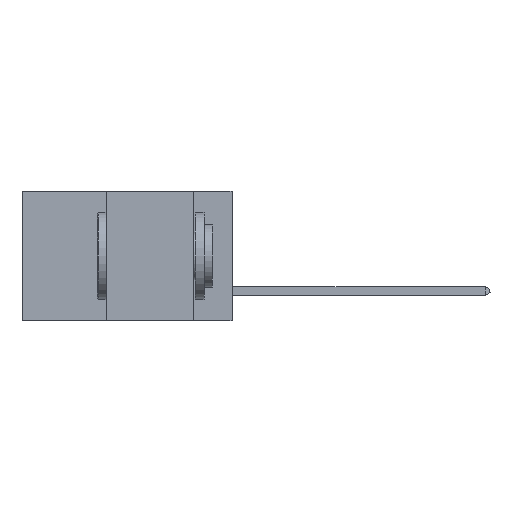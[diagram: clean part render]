
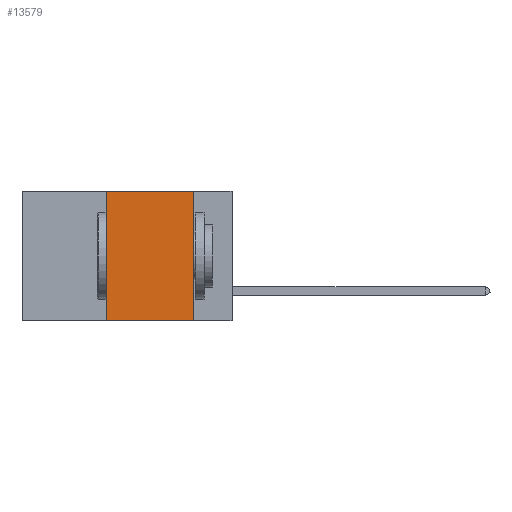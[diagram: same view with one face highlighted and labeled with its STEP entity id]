
A CAD part, left-side view. The second image highlights one B-rep face of the part: STEP entity #13579.
In plain terms, the highlighted planar face has unit normal (-1, 0, 0).
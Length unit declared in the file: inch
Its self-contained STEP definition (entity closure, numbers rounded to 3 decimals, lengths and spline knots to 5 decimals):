
#772 = VECTOR ( 'NONE', #7230, 39.37008 ) ;
#856 = EDGE_CURVE ( 'NONE', #14611, #11134, #8960, .T. ) ;
#1197 = VECTOR ( 'NONE', #9243, 39.37008 ) ;
#1568 = CARTESIAN_POINT ( 'NONE',  ( 0., 0.36, 0. ) ) ;
#1757 = CARTESIAN_POINT ( 'NONE',  ( 0., 0.36, -0.37 ) ) ;
#3604 = ORIENTED_EDGE ( 'NONE', *, *, #4131, .F. ) ;
#4131 = EDGE_CURVE ( 'NONE', #13491, #6629, #10320, .T. ) ;
#4282 = CARTESIAN_POINT ( 'NONE',  ( 0., 0.11, 0. ) ) ;
#4395 = CARTESIAN_POINT ( 'NONE',  ( 0., 0.6, -0.37 ) ) ;
#5053 = DIRECTION ( 'NONE',  ( 0., 0., -1. ) ) ;
#5174 = PLANE ( 'NONE',  #9892 ) ;
#5248 = LINE ( 'NONE', #4395, #8461 ) ;
#6492 = CARTESIAN_POINT ( 'NONE',  ( 0., 0.11, -0.37 ) ) ;
#6629 = VERTEX_POINT ( 'NONE', #1568 ) ;
#7043 = ORIENTED_EDGE ( 'NONE', *, *, #856, .F. ) ;
#7155 = EDGE_LOOP ( 'NONE', ( #7043, #13003, #3604, #12993 ) ) ;
#7230 = DIRECTION ( 'NONE',  ( 0., 0., 1. ) ) ;
#7379 = EDGE_CURVE ( 'NONE', #6629, #14611, #14307, .T. ) ;
#7556 = CARTESIAN_POINT ( 'NONE',  ( 0., 0.6, 0. ) ) ;
#8047 = FACE_OUTER_BOUND ( 'NONE', #7155, .T. ) ;
#8246 = DIRECTION ( 'NONE',  ( 0., 0., -1. ) ) ;
#8461 = VECTOR ( 'NONE', #15324, 39.37008 ) ;
#8960 = LINE ( 'NONE', #11855, #14027 ) ;
#9243 = DIRECTION ( 'NONE',  ( 0., -1., 0. ) ) ;
#9841 = CARTESIAN_POINT ( 'NONE',  ( 0., 0.6, 0. ) ) ;
#9892 = AXIS2_PLACEMENT_3D ( 'NONE', #7556, #11086, #5053 ) ;
#10320 = LINE ( 'NONE', #14398, #772 ) ;
#11086 = DIRECTION ( 'NONE',  ( 1., 0., 0. ) ) ;
#11134 = VERTEX_POINT ( 'NONE', #6492 ) ;
#11855 = CARTESIAN_POINT ( 'NONE',  ( 0., 0.11, 0. ) ) ;
#12069 = EDGE_CURVE ( 'NONE', #13491, #11134, #5248, .T. ) ;
#12993 = ORIENTED_EDGE ( 'NONE', *, *, #12069, .T. ) ;
#13003 = ORIENTED_EDGE ( 'NONE', *, *, #7379, .F. ) ;
#13491 = VERTEX_POINT ( 'NONE', #1757 ) ;
#13579 = ADVANCED_FACE ( 'NONE', ( #8047 ), #5174, .F. ) ;
#14027 = VECTOR ( 'NONE', #8246, 39.37008 ) ;
#14307 = LINE ( 'NONE', #9841, #1197 ) ;
#14398 = CARTESIAN_POINT ( 'NONE',  ( 0., 0.36, 0. ) ) ;
#14611 = VERTEX_POINT ( 'NONE', #4282 ) ;
#15324 = DIRECTION ( 'NONE',  ( 0., -1., 0. ) ) ;
